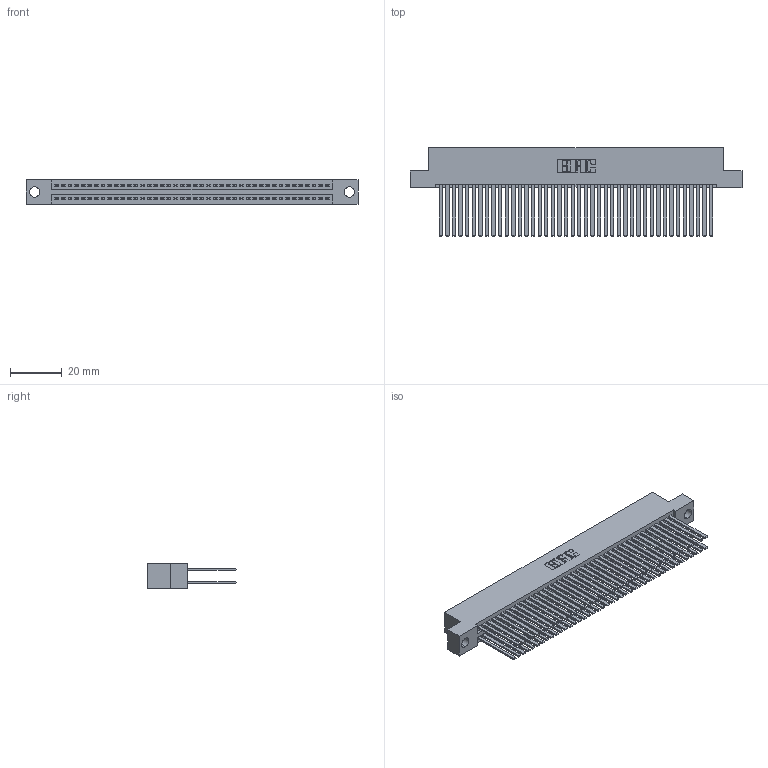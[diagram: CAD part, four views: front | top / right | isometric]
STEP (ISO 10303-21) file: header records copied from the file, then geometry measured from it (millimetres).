
FILE_DESCRIPTION (( 'STEP AP203' ), '1' );
FILE_NAME ('395-084-544-204.STEP', '2021-06-17T08:23:26', ( '' ), ( '' ), 'SwSTEP 2.0', 'SolidWorks 2020', '' );
FILE_SCHEMA (( 'CONFIG_CONTROL_DESIGN' ));
Length unit declared in the file: inch
Products named in the file (3): 345-292-001_345-293-144; 395-084-544-204; 345 Part_Flush Mounting Lugs - 0.156 Dia-TI
Assembly tree (85 placements, depth 2):
  395-084-544-204
    345 Part_Flush Mounting Lugs - 0.156 Dia-TI
    345-292-001_345-293-144  x84
Bounding box: 127.89 x 33.96 x 9.4 mm (x, y, z)
Volume: 13494.8 mm3; surface area: 23250.5 mm2
Topology: 85 solids, 85 shells, 3836 faces, 11381 edges, 7474 vertices
Faces by surface type: plane 2530, cylinder 1306
Entity records: 33189 total; most frequent: CARTESIAN_POINT 5566, ORIENTED_EDGE 5498, DIRECTION 4905, EDGE_CURVE 2749, LINE 2453, VECTOR 2453, VERTEX_POINT 1830, AXIS2_PLACEMENT_3D 1226
